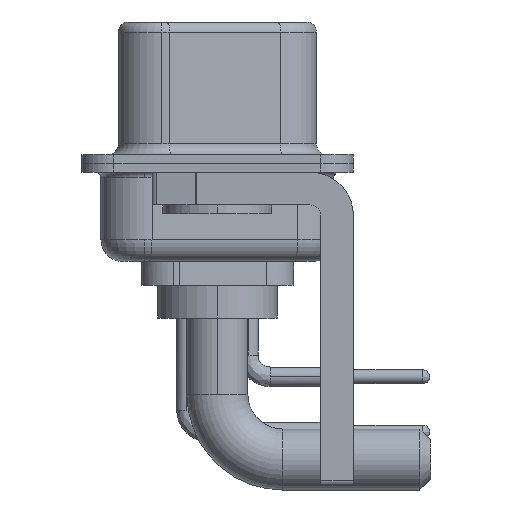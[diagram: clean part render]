
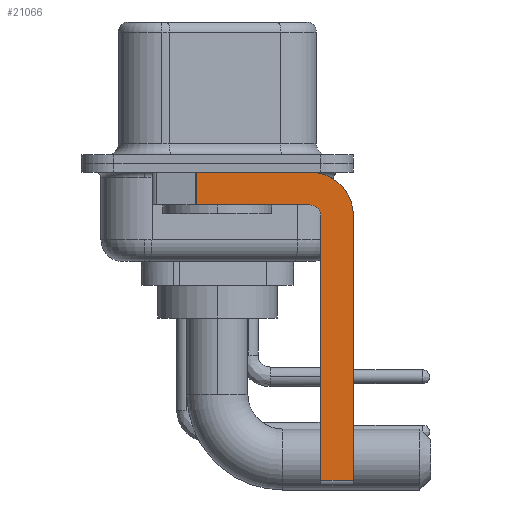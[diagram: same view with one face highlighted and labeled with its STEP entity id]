
A CAD part, left-side view. The second image highlights one B-rep face of the part: STEP entity #21066.
In plain terms, the highlighted planar face has unit normal (-1, 0, 0).
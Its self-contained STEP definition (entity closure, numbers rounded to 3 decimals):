
#118 = CIRCLE ( 'NONE', #2358, 2. ) ;
#437 = VECTOR ( 'NONE', #11657, 1000. ) ;
#1281 = LINE ( 'NONE', #8765, #8268 ) ;
#1347 = DIRECTION ( 'NONE',  ( 0., -1., 0. ) ) ;
#1486 = EDGE_CURVE ( 'NONE', #5965, #1839, #19496, .T. ) ;
#1517 = CARTESIAN_POINT ( 'NONE',  ( -2.9, -6.25, -2.4 ) ) ;
#1839 = VERTEX_POINT ( 'NONE', #15388 ) ;
#2045 = DIRECTION ( 'NONE',  ( 1., 0., 0. ) ) ;
#2055 = ORIENTED_EDGE ( 'NONE', *, *, #23121, .F. ) ;
#2166 = DIRECTION ( 'NONE',  ( 0., 0., -1. ) ) ;
#2358 = AXIS2_PLACEMENT_3D ( 'NONE', #7194, #2045, #2166 ) ;
#2409 = CARTESIAN_POINT ( 'NONE',  ( -2.9, -4.25, -0.4 ) ) ;
#3033 = CARTESIAN_POINT ( 'NONE',  ( -2.9, -6.25, -14.55 ) ) ;
#3838 = VERTEX_POINT ( 'NONE', #16716 ) ;
#3925 = CARTESIAN_POINT ( 'NONE',  ( -2.9, 3., -0.4 ) ) ;
#4896 = CIRCLE ( 'NONE', #9392, 0.5 ) ;
#5097 = LINE ( 'NONE', #12141, #15584 ) ;
#5965 = VERTEX_POINT ( 'NONE', #11721 ) ;
#6208 = ORIENTED_EDGE ( 'NONE', *, *, #10041, .F. ) ;
#6374 = VERTEX_POINT ( 'NONE', #19823 ) ;
#7152 = DIRECTION ( 'NONE',  ( 0., 0., 1. ) ) ;
#7194 = CARTESIAN_POINT ( 'NONE',  ( -2.9, -4.25, -2.4 ) ) ;
#7682 = VECTOR ( 'NONE', #7152, 1000. ) ;
#8268 = VECTOR ( 'NONE', #22890, 1000. ) ;
#8309 = DIRECTION ( 'NONE',  ( -1., 0., 0. ) ) ;
#8765 = CARTESIAN_POINT ( 'NONE',  ( -2.9, 0.978, -1.9 ) ) ;
#8906 = CARTESIAN_POINT ( 'NONE',  ( -2.9, 0.978, -0.4 ) ) ;
#9187 = EDGE_CURVE ( 'NONE', #1839, #6374, #4896, .T. ) ;
#9196 = VERTEX_POINT ( 'NONE', #3033 ) ;
#9232 = EDGE_CURVE ( 'NONE', #18683, #21743, #1281, .T. ) ;
#9392 = AXIS2_PLACEMENT_3D ( 'NONE', #13846, #8309, #19351 ) ;
#9567 = ORIENTED_EDGE ( 'NONE', *, *, #9232, .T. ) ;
#10041 = EDGE_CURVE ( 'NONE', #6374, #21743, #22593, .T. ) ;
#10852 = EDGE_CURVE ( 'NONE', #3838, #9196, #12779, .T. ) ;
#10975 = VECTOR ( 'NONE', #15968, 1000. ) ;
#11657 = DIRECTION ( 'NONE',  ( 0., 1., 0. ) ) ;
#11721 = CARTESIAN_POINT ( 'NONE',  ( -2.9, -4.75, -14.55 ) ) ;
#11922 = EDGE_CURVE ( 'NONE', #18683, #13709, #14510, .T. ) ;
#11994 = DIRECTION ( 'NONE',  ( 1., 0., 0. ) ) ;
#12141 = CARTESIAN_POINT ( 'NONE',  ( -2.9, -4.25, -14.55 ) ) ;
#12367 = CARTESIAN_POINT ( 'NONE',  ( -2.9, 0.978, -1.9 ) ) ;
#12779 = LINE ( 'NONE', #1517, #10975 ) ;
#12872 = VECTOR ( 'NONE', #22012, 1000. ) ;
#13241 = ORIENTED_EDGE ( 'NONE', *, *, #9187, .F. ) ;
#13709 = VERTEX_POINT ( 'NONE', #2409 ) ;
#13763 = PLANE ( 'NONE',  #22578 ) ;
#13846 = CARTESIAN_POINT ( 'NONE',  ( -2.9, -4.25, -2.4 ) ) ;
#13878 = CARTESIAN_POINT ( 'NONE',  ( -2.9, -4.25, -2.4 ) ) ;
#14510 = LINE ( 'NONE', #3925, #12872 ) ;
#15087 = EDGE_CURVE ( 'NONE', #5965, #9196, #5097, .T. ) ;
#15388 = CARTESIAN_POINT ( 'NONE',  ( -2.9, -4.75, -2.4 ) ) ;
#15584 = VECTOR ( 'NONE', #1347, 1000. ) ;
#15968 = DIRECTION ( 'NONE',  ( 0., 0., -1. ) ) ;
#16460 = ORIENTED_EDGE ( 'NONE', *, *, #15087, .T. ) ;
#16716 = CARTESIAN_POINT ( 'NONE',  ( -2.9, -6.25, -2.4 ) ) ;
#17067 = ORIENTED_EDGE ( 'NONE', *, *, #1486, .F. ) ;
#17202 = EDGE_LOOP ( 'NONE', ( #20672, #9567, #6208, #13241, #17067, #16460, #20732, #2055 ) ) ;
#17302 = CARTESIAN_POINT ( 'NONE',  ( -2.9, -4.25, -1.9 ) ) ;
#18683 = VERTEX_POINT ( 'NONE', #8906 ) ;
#19151 = CARTESIAN_POINT ( 'NONE',  ( -2.9, -4.75, -14.8 ) ) ;
#19269 = DIRECTION ( 'NONE',  ( 0., 0., -1. ) ) ;
#19351 = DIRECTION ( 'NONE',  ( 0., 0., 1. ) ) ;
#19496 = LINE ( 'NONE', #19151, #7682 ) ;
#19823 = CARTESIAN_POINT ( 'NONE',  ( -2.9, -4.25, -1.9 ) ) ;
#20672 = ORIENTED_EDGE ( 'NONE', *, *, #11922, .F. ) ;
#20686 = FACE_OUTER_BOUND ( 'NONE', #17202, .T. ) ;
#20732 = ORIENTED_EDGE ( 'NONE', *, *, #10852, .F. ) ;
#21066 = ADVANCED_FACE ( 'NONE', ( #20686 ), #13763, .F. ) ;
#21743 = VERTEX_POINT ( 'NONE', #12367 ) ;
#22012 = DIRECTION ( 'NONE',  ( 0., -1., 0. ) ) ;
#22578 = AXIS2_PLACEMENT_3D ( 'NONE', #13878, #11994, #19269 ) ;
#22593 = LINE ( 'NONE', #17302, #437 ) ;
#22890 = DIRECTION ( 'NONE',  ( 0., 0., -1. ) ) ;
#23121 = EDGE_CURVE ( 'NONE', #13709, #3838, #118, .T. ) ;
